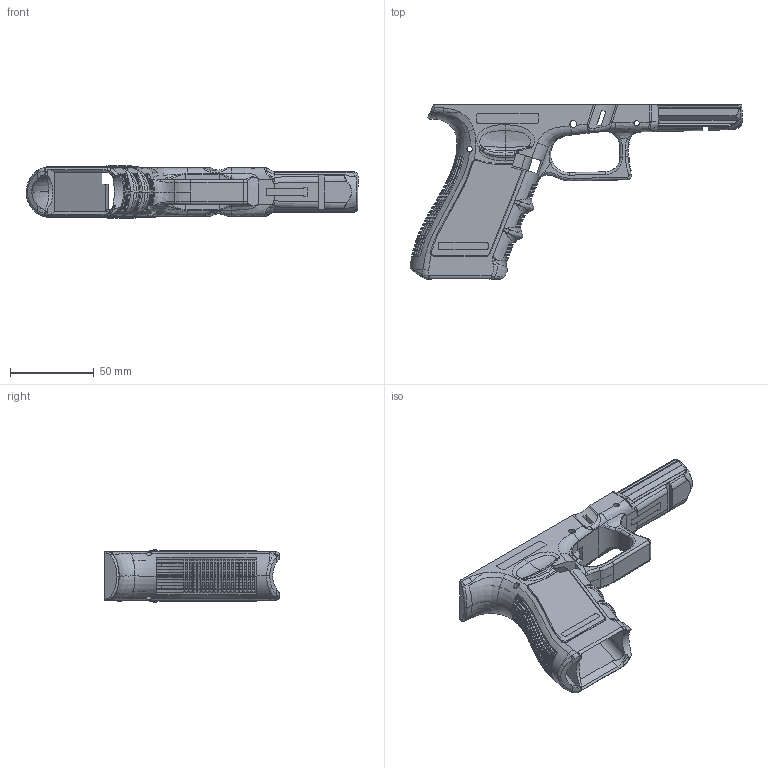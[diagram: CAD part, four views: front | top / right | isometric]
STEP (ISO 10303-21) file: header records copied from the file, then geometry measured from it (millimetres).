
FILE_DESCRIPTION(/* description */ (''),/* implementation_level */ '2;1');
FILE_NAME(/* name */ 'PrintYour2A G17.2.step',/* time_stamp */ '2020-09-26T15:42:14-05:00',/* author */ (''),/* organization */ (''),/* preprocessor_version */ 'ST-DEVELOPER v18.1',/* originating_system */ 'Autodesk Translation Framework v9.3.0.1241',/* authorisation */ '');
FILE_SCHEMA (('AUTOMOTIVE_DESIGN { 1 0 10303 214 3 1 1 }'));
Products named in the file (1): PrintYour2A G17
Bounding box: 197.79 x 104 x 31.4 mm (x, y, z)
Volume: 85929.3 mm3; surface area: 52725.4 mm2
Topology: 1 solids, 1 shells, 2131 faces, 6096 edges, 3947 vertices
Faces by surface type: bspline 911, plane 869, cylinder 328, torus 16, cone 5, sphere 2
Full cylindrical faces by diameter (mm): 1.5 x2, 3.225 x2, 3.25 x2
Entity records: 185065 total; most frequent: CARTESIAN_POINT 136654, ORIENTED_EDGE 12182, DIRECTION 7196, EDGE_CURVE 6091, VERTEX_POINT 3956, LINE 2522, VECTOR 2522, B_SPLINE_CURVE_WITH_KNOTS 2450
